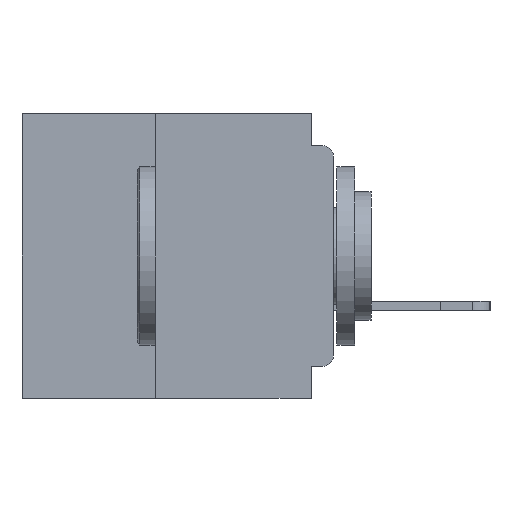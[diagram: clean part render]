
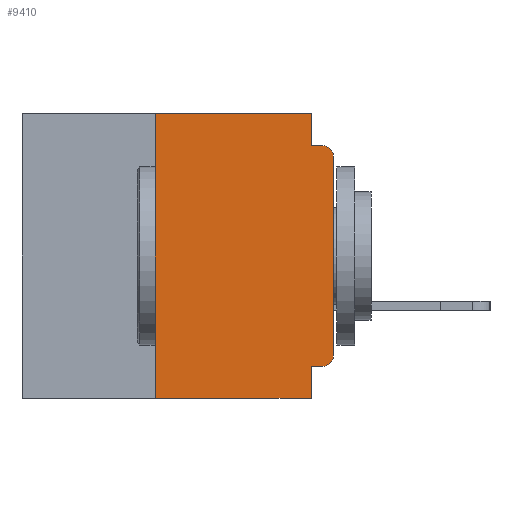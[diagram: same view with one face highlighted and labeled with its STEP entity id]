
A CAD part, left-side view. The second image highlights one B-rep face of the part: STEP entity #9410.
In plain terms, the highlighted planar face has unit normal (-1, 0, 0).
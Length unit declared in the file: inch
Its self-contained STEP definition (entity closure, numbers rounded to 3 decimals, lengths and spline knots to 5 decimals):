
#407 = DIRECTION ( 'NONE',  ( 0., -1., 0. ) ) ;
#1850 = CARTESIAN_POINT ( 'NONE',  ( 0., 0.015, -0.34 ) ) ;
#4279 = DIRECTION ( 'NONE',  ( 0., 0., -1. ) ) ;
#4343 = EDGE_LOOP ( 'NONE', ( #53165, #11425, #29183, #47284, #26512, #54225, #52661, #43499, #33043, #13908 ) ) ;
#6533 = DIRECTION ( 'NONE',  ( 0., 0., -1. ) ) ;
#7447 = EDGE_CURVE ( 'NONE', #45360, #51635, #51158, .T. ) ;
#9130 = CARTESIAN_POINT ( 'NONE',  ( 0., 0.031, 0. ) ) ;
#9410 = ADVANCED_FACE ( 'NONE', ( #23981 ), #29867, .F. ) ;
#9743 = CARTESIAN_POINT ( 'NONE',  ( 0., 0., -0.045 ) ) ;
#9764 = LINE ( 'NONE', #58572, #44457 ) ;
#10705 = DIRECTION ( 'NONE',  ( 0., 0., 1. ) ) ;
#11425 = ORIENTED_EDGE ( 'NONE', *, *, #43761, .T. ) ;
#13106 = EDGE_CURVE ( 'NONE', #45663, #17461, #49979, .T. ) ;
#13565 = AXIS2_PLACEMENT_3D ( 'NONE', #1850, #33751, #6533 ) ;
#13908 = ORIENTED_EDGE ( 'NONE', *, *, #57520, .T. ) ;
#14054 = CARTESIAN_POINT ( 'NONE',  ( 0., 0.031, 0. ) ) ;
#14567 = EDGE_CURVE ( 'NONE', #58583, #53420, #54102, .T. ) ;
#16308 = LINE ( 'NONE', #51469, #26887 ) ;
#16403 = DIRECTION ( 'NONE',  ( 0., 0., -1. ) ) ;
#17028 = CIRCLE ( 'NONE', #39269, 0.015 ) ;
#17411 = CARTESIAN_POINT ( 'NONE',  ( 0., 0.437, -0.4 ) ) ;
#17461 = VERTEX_POINT ( 'NONE', #55970 ) ;
#18097 = DIRECTION ( 'NONE',  ( 0., -1., 0. ) ) ;
#18981 = EDGE_CURVE ( 'NONE', #37205, #29100, #34304, .T. ) ;
#20531 = CARTESIAN_POINT ( 'NONE',  ( 0., 0.015, -0.355 ) ) ;
#21078 = DIRECTION ( 'NONE',  ( 0., 0., 1. ) ) ;
#22150 = EDGE_CURVE ( 'NONE', #17461, #46278, #26060, .T. ) ;
#22694 = CARTESIAN_POINT ( 'NONE',  ( 0., 0.015, -0.06 ) ) ;
#23981 = FACE_OUTER_BOUND ( 'NONE', #4343, .T. ) ;
#24148 = CARTESIAN_POINT ( 'NONE',  ( 0., 0., -0.06 ) ) ;
#24197 = AXIS2_PLACEMENT_3D ( 'NONE', #52450, #43562, #16403 ) ;
#25481 = CARTESIAN_POINT ( 'NONE',  ( 0., 0.25, -0.4 ) ) ;
#25807 = VECTOR ( 'NONE', #41211, 39.37008 ) ;
#26060 = LINE ( 'NONE', #9743, #47384 ) ;
#26512 = ORIENTED_EDGE ( 'NONE', *, *, #56617, .F. ) ;
#26887 = VECTOR ( 'NONE', #10705, 39.37008 ) ;
#27277 = DIRECTION ( 'NONE',  ( 0., 0., -1. ) ) ;
#29100 = VERTEX_POINT ( 'NONE', #30405 ) ;
#29183 = ORIENTED_EDGE ( 'NONE', *, *, #22150, .F. ) ;
#29867 = PLANE ( 'NONE',  #24197 ) ;
#30405 = CARTESIAN_POINT ( 'NONE',  ( 0., 0.031, -0.4 ) ) ;
#31082 = DIRECTION ( 'NONE',  ( 0., -1., 0. ) ) ;
#32776 = DIRECTION ( 'NONE',  ( 0., 1., 0. ) ) ;
#32855 = VECTOR ( 'NONE', #31082, 39.37008 ) ;
#33043 = ORIENTED_EDGE ( 'NONE', *, *, #7447, .F. ) ;
#33077 = LINE ( 'NONE', #54161, #55666 ) ;
#33751 = DIRECTION ( 'NONE',  ( -1., 0., 0. ) ) ;
#34304 = LINE ( 'NONE', #17411, #32855 ) ;
#36166 = CARTESIAN_POINT ( 'NONE',  ( 0., 0.25, 0. ) ) ;
#37145 = CARTESIAN_POINT ( 'NONE',  ( 0., 0., -0.355 ) ) ;
#37205 = VERTEX_POINT ( 'NONE', #25481 ) ;
#38583 = VERTEX_POINT ( 'NONE', #36166 ) ;
#39144 = VECTOR ( 'NONE', #32776, 39.37008 ) ;
#39269 = AXIS2_PLACEMENT_3D ( 'NONE', #22694, #54422, #27277 ) ;
#41211 = DIRECTION ( 'NONE',  ( 0., 0., -1. ) ) ;
#43499 = ORIENTED_EDGE ( 'NONE', *, *, #55941, .F. ) ;
#43559 = CIRCLE ( 'NONE', #13565, 0.015 ) ;
#43562 = DIRECTION ( 'NONE',  ( 1., 0., 0. ) ) ;
#43761 = EDGE_CURVE ( 'NONE', #53420, #46278, #17028, .T. ) ;
#43966 = EDGE_CURVE ( 'NONE', #37205, #38583, #16308, .T. ) ;
#44093 = CARTESIAN_POINT ( 'NONE',  ( 0., 0., -0.34 ) ) ;
#44457 = VECTOR ( 'NONE', #4279, 39.37008 ) ;
#45360 = VERTEX_POINT ( 'NONE', #20531 ) ;
#45663 = VERTEX_POINT ( 'NONE', #9130 ) ;
#46278 = VERTEX_POINT ( 'NONE', #49627 ) ;
#47284 = ORIENTED_EDGE ( 'NONE', *, *, #13106, .F. ) ;
#47384 = VECTOR ( 'NONE', #407, 39.37008 ) ;
#48642 = CARTESIAN_POINT ( 'NONE',  ( 0., 0.031, -0.355 ) ) ;
#49627 = CARTESIAN_POINT ( 'NONE',  ( 0., 0.015, -0.045 ) ) ;
#49979 = LINE ( 'NONE', #14054, #25807 ) ;
#51158 = LINE ( 'NONE', #37145, #39144 ) ;
#51292 = VECTOR ( 'NONE', #21078, 39.37008 ) ;
#51469 = CARTESIAN_POINT ( 'NONE',  ( 0., 0.25, -0.4 ) ) ;
#51635 = VERTEX_POINT ( 'NONE', #48642 ) ;
#52450 = CARTESIAN_POINT ( 'NONE',  ( 0., 0.437, 0. ) ) ;
#52661 = ORIENTED_EDGE ( 'NONE', *, *, #18981, .T. ) ;
#52819 = CARTESIAN_POINT ( 'NONE',  ( 0., 0., 0. ) ) ;
#53165 = ORIENTED_EDGE ( 'NONE', *, *, #14567, .T. ) ;
#53420 = VERTEX_POINT ( 'NONE', #24148 ) ;
#54102 = LINE ( 'NONE', #52819, #51292 ) ;
#54161 = CARTESIAN_POINT ( 'NONE',  ( 0., 0.437, 0. ) ) ;
#54225 = ORIENTED_EDGE ( 'NONE', *, *, #43966, .F. ) ;
#54422 = DIRECTION ( 'NONE',  ( -1., 0., 0. ) ) ;
#55666 = VECTOR ( 'NONE', #18097, 39.37008 ) ;
#55941 = EDGE_CURVE ( 'NONE', #51635, #29100, #9764, .T. ) ;
#55970 = CARTESIAN_POINT ( 'NONE',  ( 0., 0.031, -0.045 ) ) ;
#56617 = EDGE_CURVE ( 'NONE', #38583, #45663, #33077, .T. ) ;
#57520 = EDGE_CURVE ( 'NONE', #45360, #58583, #43559, .T. ) ;
#58572 = CARTESIAN_POINT ( 'NONE',  ( 0., 0.031, -0.4 ) ) ;
#58583 = VERTEX_POINT ( 'NONE', #44093 ) ;
